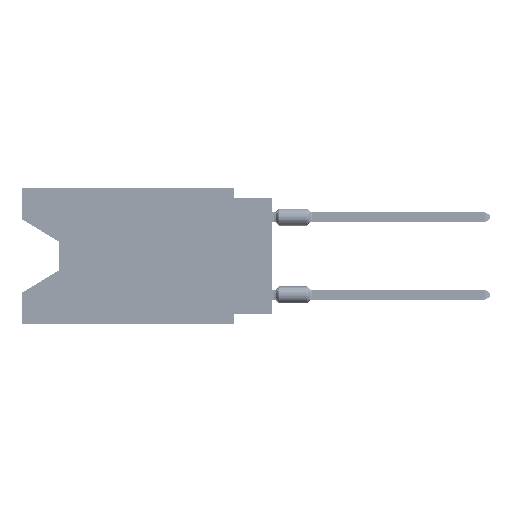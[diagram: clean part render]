
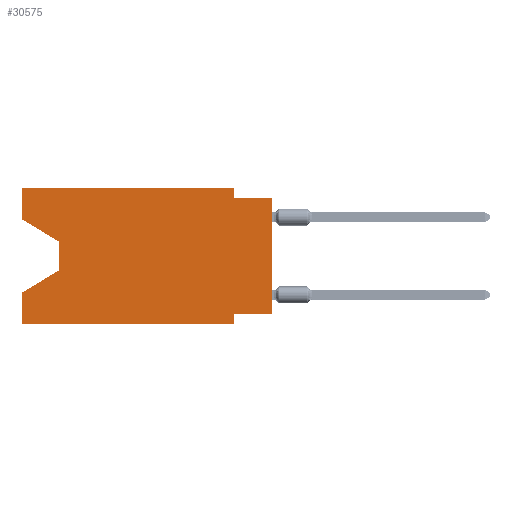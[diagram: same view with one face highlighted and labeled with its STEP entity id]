
A CAD part, left-side view. The second image highlights one B-rep face of the part: STEP entity #30575.
In plain terms, the highlighted planar face has unit normal (-1, 0, 0).
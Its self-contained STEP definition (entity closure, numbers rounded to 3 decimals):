
#1848 = CARTESIAN_POINT ( 'NONE',  ( 0., 16.383, -6.852 ) ) ;
#3681 = VERTEX_POINT ( 'NONE', #24723 ) ;
#4502 = ORIENTED_EDGE ( 'NONE', *, *, #55470, .T. ) ;
#5572 = CARTESIAN_POINT ( 'NONE',  ( 0., 2.54, -8.255 ) ) ;
#5614 = VERTEX_POINT ( 'NONE', #67726 ) ;
#6419 = ORIENTED_EDGE ( 'NONE', *, *, #56539, .F. ) ;
#6899 = EDGE_CURVE ( 'NONE', #78351, #89768, #88993, .T. ) ;
#7806 = DIRECTION ( 'NONE',  ( 0., 0.855, -0.519 ) ) ;
#7945 = CARTESIAN_POINT ( 'NONE',  ( 0., 16.383, -2.038 ) ) ;
#8499 = CARTESIAN_POINT ( 'NONE',  ( 0., 13.97, -5.385 ) ) ;
#9047 = CARTESIAN_POINT ( 'NONE',  ( 0., 16.383, -8.89 ) ) ;
#9603 = VERTEX_POINT ( 'NONE', #1848 ) ;
#10929 = LINE ( 'NONE', #55955, #35457 ) ;
#13015 = LINE ( 'NONE', #51392, #98480 ) ;
#13330 = DIRECTION ( 'NONE',  ( 1., 0., 0. ) ) ;
#15958 = VECTOR ( 'NONE', #115426, 1000. ) ;
#16730 = DIRECTION ( 'NONE',  ( 0., 0., 1. ) ) ;
#18253 = VECTOR ( 'NONE', #7806, 1000. ) ;
#19414 = VERTEX_POINT ( 'NONE', #9047 ) ;
#22777 = EDGE_CURVE ( 'NONE', #3681, #112817, #113350, .T. ) ;
#24060 = VECTOR ( 'NONE', #35286, 1000. ) ;
#24457 = VECTOR ( 'NONE', #108608, 1000. ) ;
#24723 = CARTESIAN_POINT ( 'NONE',  ( 0., 13.97, -3.505 ) ) ;
#30575 = ADVANCED_FACE ( 'NONE', ( #110164 ), #48738, .F. ) ;
#31276 = EDGE_CURVE ( 'NONE', #19414, #9603, #98952, .T. ) ;
#32510 = ORIENTED_EDGE ( 'NONE', *, *, #54926, .T. ) ;
#32554 = ORIENTED_EDGE ( 'NONE', *, *, #73465, .F. ) ;
#33984 = ORIENTED_EDGE ( 'NONE', *, *, #102667, .T. ) ;
#35286 = DIRECTION ( 'NONE',  ( 0., 0., 1. ) ) ;
#35457 = VECTOR ( 'NONE', #59923, 1000. ) ;
#36379 = ORIENTED_EDGE ( 'NONE', *, *, #6899, .F. ) ;
#37543 = CARTESIAN_POINT ( 'NONE',  ( 0., 16.383, 0. ) ) ;
#38657 = CARTESIAN_POINT ( 'NONE',  ( 0., 0., -8.255 ) ) ;
#39553 = CARTESIAN_POINT ( 'NONE',  ( 0., 13.97, -3.505 ) ) ;
#39745 = DIRECTION ( 'NONE',  ( 0., 0., -1. ) ) ;
#41503 = VERTEX_POINT ( 'NONE', #59017 ) ;
#42198 = DIRECTION ( 'NONE',  ( 0., -1., 0. ) ) ;
#42949 = ORIENTED_EDGE ( 'NONE', *, *, #52204, .T. ) ;
#43096 = CARTESIAN_POINT ( 'NONE',  ( 0., 0., 0. ) ) ;
#43547 = LINE ( 'NONE', #80147, #96303 ) ;
#43997 = CARTESIAN_POINT ( 'NONE',  ( 0., 2.54, 0. ) ) ;
#44789 = CARTESIAN_POINT ( 'NONE',  ( 0., 0., -0.635 ) ) ;
#48350 = ORIENTED_EDGE ( 'NONE', *, *, #53351, .F. ) ;
#48738 = PLANE ( 'NONE',  #64058 ) ;
#51392 = CARTESIAN_POINT ( 'NONE',  ( 0., 16.383, 0. ) ) ;
#52204 = EDGE_CURVE ( 'NONE', #19414, #5614, #43547, .T. ) ;
#53351 = EDGE_CURVE ( 'NONE', #97610, #5614, #107175, .T. ) ;
#54926 = EDGE_CURVE ( 'NONE', #112817, #9603, #71454, .T. ) ;
#55470 = EDGE_CURVE ( 'NONE', #78952, #89768, #61677, .T. ) ;
#55955 = CARTESIAN_POINT ( 'NONE',  ( 0., 16.383, 0. ) ) ;
#56539 = EDGE_CURVE ( 'NONE', #95145, #79229, #10929, .T. ) ;
#57491 = ORIENTED_EDGE ( 'NONE', *, *, #31276, .F. ) ;
#58832 = ORIENTED_EDGE ( 'NONE', *, *, #64205, .F. ) ;
#59017 = CARTESIAN_POINT ( 'NONE',  ( 0., 2.54, 0. ) ) ;
#59462 = ORIENTED_EDGE ( 'NONE', *, *, #106839, .F. ) ;
#59923 = DIRECTION ( 'NONE',  ( 0., 0., 1. ) ) ;
#60762 = CARTESIAN_POINT ( 'NONE',  ( 0., 16.383, 0. ) ) ;
#60785 = LINE ( 'NONE', #43997, #15958 ) ;
#61677 = LINE ( 'NONE', #43096, #24060 ) ;
#62920 = CARTESIAN_POINT ( 'NONE',  ( 0., 16.383, 0. ) ) ;
#64058 = AXIS2_PLACEMENT_3D ( 'NONE', #37543, #13330, #39745 ) ;
#64205 = EDGE_CURVE ( 'NONE', #79229, #41503, #13015, .T. ) ;
#67726 = CARTESIAN_POINT ( 'NONE',  ( 0., 2.54, -8.89 ) ) ;
#68027 = CARTESIAN_POINT ( 'NONE',  ( 0., 0., -0.635 ) ) ;
#71454 = LINE ( 'NONE', #89444, #18253 ) ;
#73210 = CARTESIAN_POINT ( 'NONE',  ( 0., 0., -8.255 ) ) ;
#73465 = EDGE_CURVE ( 'NONE', #78952, #97610, #109800, .T. ) ;
#75397 = VECTOR ( 'NONE', #89758, 1000. ) ;
#77592 = VECTOR ( 'NONE', #16730, 1000. ) ;
#78351 = VERTEX_POINT ( 'NONE', #79819 ) ;
#78952 = VERTEX_POINT ( 'NONE', #38657 ) ;
#79229 = VERTEX_POINT ( 'NONE', #60762 ) ;
#79819 = CARTESIAN_POINT ( 'NONE',  ( 0., 2.54, -0.635 ) ) ;
#80147 = CARTESIAN_POINT ( 'NONE',  ( 0., 16.383, -8.89 ) ) ;
#82366 = VECTOR ( 'NONE', #117780, 1000. ) ;
#84583 = DIRECTION ( 'NONE',  ( 0., 0., -1. ) ) ;
#88993 = LINE ( 'NONE', #68027, #100782 ) ;
#89444 = CARTESIAN_POINT ( 'NONE',  ( 0., 13.97, -5.385 ) ) ;
#89758 = DIRECTION ( 'NONE',  ( 0., 0., -1. ) ) ;
#89768 = VERTEX_POINT ( 'NONE', #44789 ) ;
#90360 = CARTESIAN_POINT ( 'NONE',  ( 0., 2.54, -8.89 ) ) ;
#95145 = VERTEX_POINT ( 'NONE', #113530 ) ;
#96303 = VECTOR ( 'NONE', #116746, 1000. ) ;
#97610 = VERTEX_POINT ( 'NONE', #5572 ) ;
#98480 = VECTOR ( 'NONE', #105425, 1000. ) ;
#98952 = LINE ( 'NONE', #62920, #77592 ) ;
#100782 = VECTOR ( 'NONE', #42198, 1000. ) ;
#101190 = ORIENTED_EDGE ( 'NONE', *, *, #22777, .T. ) ;
#102667 = EDGE_CURVE ( 'NONE', #95145, #3681, #108767, .T. ) ;
#103074 = VECTOR ( 'NONE', #84583, 1000. ) ;
#105425 = DIRECTION ( 'NONE',  ( 0., -1., 0. ) ) ;
#106839 = EDGE_CURVE ( 'NONE', #41503, #78351, #60785, .T. ) ;
#107175 = LINE ( 'NONE', #90360, #75397 ) ;
#108608 = DIRECTION ( 'NONE',  ( 0., 1., 0. ) ) ;
#108767 = LINE ( 'NONE', #7945, #82366 ) ;
#109800 = LINE ( 'NONE', #73210, #24457 ) ;
#110164 = FACE_OUTER_BOUND ( 'NONE', #116236, .T. ) ;
#112817 = VERTEX_POINT ( 'NONE', #8499 ) ;
#113350 = LINE ( 'NONE', #39553, #103074 ) ;
#113530 = CARTESIAN_POINT ( 'NONE',  ( 0., 16.383, -2.038 ) ) ;
#115426 = DIRECTION ( 'NONE',  ( 0., 0., -1. ) ) ;
#116236 = EDGE_LOOP ( 'NONE', ( #33984, #101190, #32510, #57491, #42949, #48350, #32554, #4502, #36379, #59462, #58832, #6419 ) ) ;
#116746 = DIRECTION ( 'NONE',  ( 0., -1., 0. ) ) ;
#117780 = DIRECTION ( 'NONE',  ( 0., -0.855, -0.519 ) ) ;
